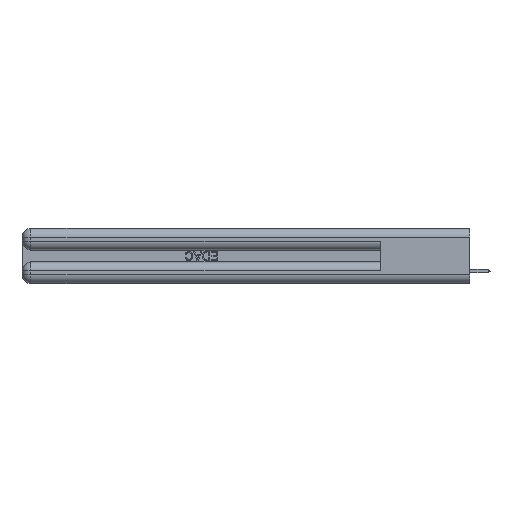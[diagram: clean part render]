
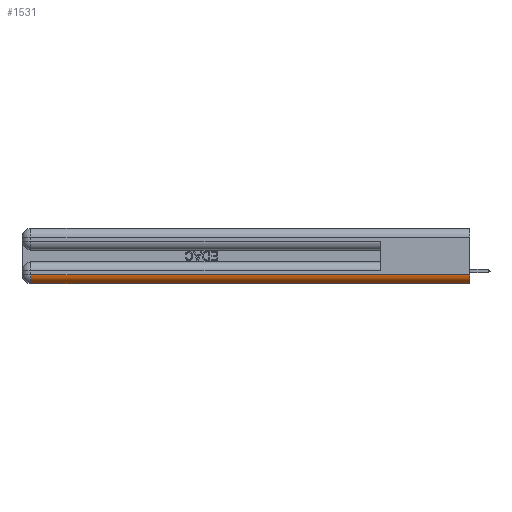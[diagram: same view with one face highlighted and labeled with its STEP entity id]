
A CAD part, left-side view. The second image highlights one B-rep face of the part: STEP entity #1531.
In plain terms, the highlighted cylindrical face has radius 1.524 mm (diameter 3.048 mm), a partial arc.
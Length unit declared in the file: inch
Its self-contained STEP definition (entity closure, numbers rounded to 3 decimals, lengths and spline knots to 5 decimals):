
#1429 = CARTESIAN_POINT ( 'NONE',  ( 0., 2.94, 0.06 ) ) ;
#1531 = ADVANCED_FACE ( 'NONE', ( #27744 ), #21043, .T. ) ;
#2521 = EDGE_CURVE ( 'NONE', #41986, #45327, #18669, .T. ) ;
#3849 = EDGE_CURVE ( 'NONE', #45327, #8256, #16932, .T. ) ;
#3922 = CARTESIAN_POINT ( 'NONE',  ( 0.06, 0., 0.06 ) ) ;
#6055 = CARTESIAN_POINT ( 'NONE',  ( 0.06, 2.94, 0. ) ) ;
#7798 = DIRECTION ( 'NONE',  ( 0., -1., 0. ) ) ;
#8256 = VERTEX_POINT ( 'NONE', #6055 ) ;
#9724 = ORIENTED_EDGE ( 'NONE', *, *, #10626, .F. ) ;
#10626 = EDGE_CURVE ( 'NONE', #43746, #41986, #33457, .T. ) ;
#12305 = CIRCLE ( 'NONE', #31799, 0.06 ) ;
#12803 = CARTESIAN_POINT ( 'NONE',  ( 0.06, 0., 0.06 ) ) ;
#13331 = CARTESIAN_POINT ( 'NONE',  ( 0.06, 2.94, 0.06 ) ) ;
#16894 = DIRECTION ( 'NONE',  ( 0., 1., 0. ) ) ;
#16932 = LINE ( 'NONE', #21293, #42634 ) ;
#18446 = CARTESIAN_POINT ( 'NONE',  ( 0., 0., 0.06 ) ) ;
#18669 = CIRCLE ( 'NONE', #22816, 0.06 ) ;
#18725 = EDGE_CURVE ( 'NONE', #8256, #43746, #12305, .T. ) ;
#21043 = CYLINDRICAL_SURFACE ( 'NONE', #39790, 0.06 ) ;
#21293 = CARTESIAN_POINT ( 'NONE',  ( 0.06, 3., 0. ) ) ;
#21874 = DIRECTION ( 'NONE',  ( 0., 1., 0. ) ) ;
#22209 = DIRECTION ( 'NONE',  ( 0., -1., 0. ) ) ;
#22816 = AXIS2_PLACEMENT_3D ( 'NONE', #3922, #7798, #40597 ) ;
#23979 = VECTOR ( 'NONE', #22209, 39.37008 ) ;
#26429 = ORIENTED_EDGE ( 'NONE', *, *, #2521, .F. ) ;
#27744 = FACE_OUTER_BOUND ( 'NONE', #38708, .T. ) ;
#31799 = AXIS2_PLACEMENT_3D ( 'NONE', #13331, #16894, #34950 ) ;
#33457 = LINE ( 'NONE', #39952, #23979 ) ;
#34950 = DIRECTION ( 'NONE',  ( 0., 0., 1. ) ) ;
#34967 = ORIENTED_EDGE ( 'NONE', *, *, #18725, .F. ) ;
#35983 = CARTESIAN_POINT ( 'NONE',  ( 0.06, 0., 0. ) ) ;
#38708 = EDGE_LOOP ( 'NONE', ( #26429, #9724, #34967, #41310 ) ) ;
#39790 = AXIS2_PLACEMENT_3D ( 'NONE', #12803, #42613, #39887 ) ;
#39887 = DIRECTION ( 'NONE',  ( 0., 0., 1. ) ) ;
#39952 = CARTESIAN_POINT ( 'NONE',  ( 0., 0., 0.06 ) ) ;
#40597 = DIRECTION ( 'NONE',  ( 0., 0., 1. ) ) ;
#41310 = ORIENTED_EDGE ( 'NONE', *, *, #3849, .F. ) ;
#41986 = VERTEX_POINT ( 'NONE', #18446 ) ;
#42613 = DIRECTION ( 'NONE',  ( 0., 1., 0. ) ) ;
#42634 = VECTOR ( 'NONE', #21874, 39.37008 ) ;
#43746 = VERTEX_POINT ( 'NONE', #1429 ) ;
#45327 = VERTEX_POINT ( 'NONE', #35983 ) ;
